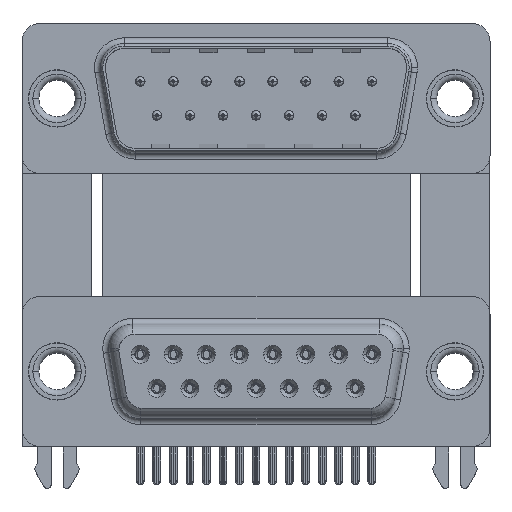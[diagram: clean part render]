
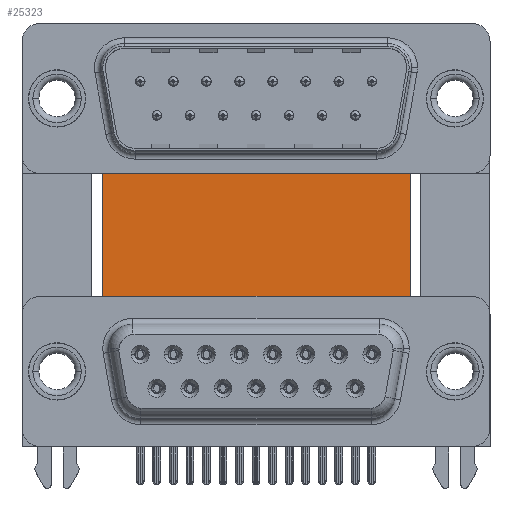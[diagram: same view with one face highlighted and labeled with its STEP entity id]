
A CAD part, top view. The second image highlights one B-rep face of the part: STEP entity #25323.
In plain terms, the highlighted planar face has unit normal (0, 0, 1).
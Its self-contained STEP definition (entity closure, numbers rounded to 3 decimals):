
#1456 = EDGE_CURVE ( 'NONE', #7083, #13791, #27085, .T. ) ;
#4264 = EDGE_CURVE ( 'NONE', #19096, #29304, #34872, .T. ) ;
#6044 = CARTESIAN_POINT ( 'NONE',  ( 3.79, 16.585, -12. ) ) ;
#6197 = PLANE ( 'NONE',  #37748 ) ;
#7083 = VERTEX_POINT ( 'NONE', #29406 ) ;
#7381 = DIRECTION ( 'NONE',  ( 0., -1., 0. ) ) ;
#9491 = CARTESIAN_POINT ( 'NONE',  ( 3.79, -3.735, -12. ) ) ;
#10746 = EDGE_CURVE ( 'NONE', #13791, #29304, #32551, .T. ) ;
#12632 = DIRECTION ( 'NONE',  ( 1., 0., 0. ) ) ;
#13791 = VERTEX_POINT ( 'NONE', #40275 ) ;
#15187 = VECTOR ( 'NONE', #33339, 1000. ) ;
#16448 = VECTOR ( 'NONE', #7381, 1000. ) ;
#19096 = VERTEX_POINT ( 'NONE', #34645 ) ;
#19838 = CARTESIAN_POINT ( 'NONE',  ( 3.79, 16.585, -12. ) ) ;
#22117 = CARTESIAN_POINT ( 'NONE',  ( 3.79, 16.585, -12. ) ) ;
#24582 = ORIENTED_EDGE ( 'NONE', *, *, #26331, .F. ) ;
#25323 = ADVANCED_FACE ( 'NONE', ( #33494 ), #6197, .F. ) ;
#26331 = EDGE_CURVE ( 'NONE', #7083, #19096, #39118, .T. ) ;
#27085 = LINE ( 'NONE', #6044, #15187 ) ;
#27851 = VECTOR ( 'NONE', #36415, 1000. ) ;
#28500 = CARTESIAN_POINT ( 'NONE',  ( 29.58, -3.735, -12. ) ) ;
#29304 = VERTEX_POINT ( 'NONE', #28500 ) ;
#29406 = CARTESIAN_POINT ( 'NONE',  ( 3.79, 16.585, -12. ) ) ;
#29541 = ORIENTED_EDGE ( 'NONE', *, *, #1456, .T. ) ;
#30889 = CARTESIAN_POINT ( 'NONE',  ( 29.58, 16.585, -12. ) ) ;
#32551 = LINE ( 'NONE', #9491, #38432 ) ;
#33339 = DIRECTION ( 'NONE',  ( 0., -1., 0. ) ) ;
#33494 = FACE_OUTER_BOUND ( 'NONE', #35327, .T. ) ;
#33716 = DIRECTION ( 'NONE',  ( -1., 0., 0. ) ) ;
#34645 = CARTESIAN_POINT ( 'NONE',  ( 29.58, 16.585, -12. ) ) ;
#34872 = LINE ( 'NONE', #30889, #16448 ) ;
#35327 = EDGE_LOOP ( 'NONE', ( #35737, #43278, #24582, #29541 ) ) ;
#35737 = ORIENTED_EDGE ( 'NONE', *, *, #10746, .T. ) ;
#36415 = DIRECTION ( 'NONE',  ( 1., 0., 0. ) ) ;
#37748 = AXIS2_PLACEMENT_3D ( 'NONE', #19838, #43783, #33716 ) ;
#38432 = VECTOR ( 'NONE', #12632, 1000. ) ;
#39118 = LINE ( 'NONE', #22117, #27851 ) ;
#40275 = CARTESIAN_POINT ( 'NONE',  ( 3.79, -3.735, -12. ) ) ;
#43278 = ORIENTED_EDGE ( 'NONE', *, *, #4264, .F. ) ;
#43783 = DIRECTION ( 'NONE',  ( 0., 0., -1. ) ) ;
